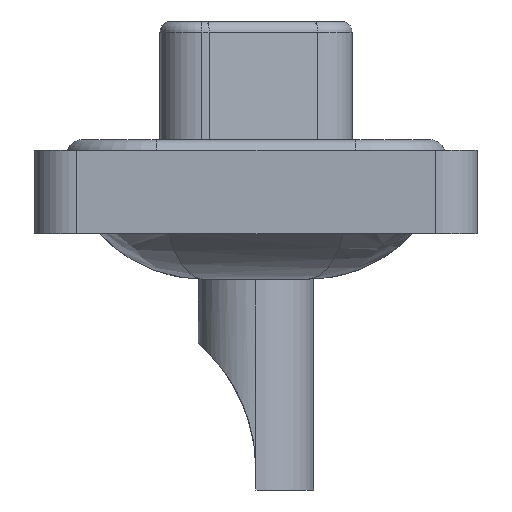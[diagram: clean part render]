
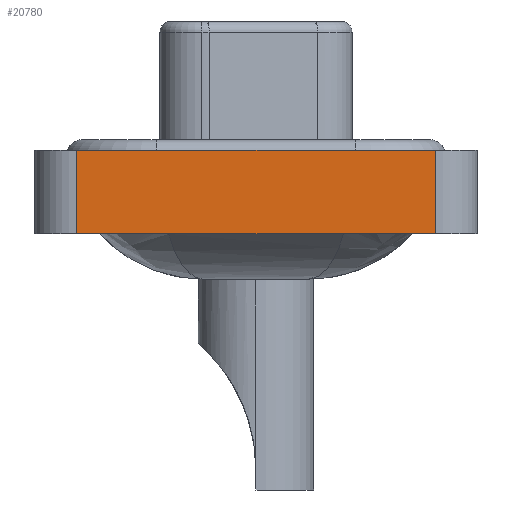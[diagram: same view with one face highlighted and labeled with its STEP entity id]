
A CAD part, left-side view. The second image highlights one B-rep face of the part: STEP entity #20780.
In plain terms, the highlighted planar face has unit normal (-1, 0, 0).
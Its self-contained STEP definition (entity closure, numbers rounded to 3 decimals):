
#815 = EDGE_LOOP ( 'NONE', ( #18101, #12877, #14945, #6495 ) ) ;
#1087 = DIRECTION ( 'NONE',  ( 0., 0., 1. ) ) ;
#1105 = VERTEX_POINT ( 'NONE', #16178 ) ;
#3852 = VERTEX_POINT ( 'NONE', #3913 ) ;
#3913 = CARTESIAN_POINT ( 'NONE',  ( -7.35, 8.55, 0.4 ) ) ;
#5101 = CARTESIAN_POINT ( 'NONE',  ( -7.35, -8.55, -3.6 ) ) ;
#5322 = DIRECTION ( 'NONE',  ( -1., 0., 0. ) ) ;
#5426 = DIRECTION ( 'NONE',  ( 0., 0., 1. ) ) ;
#6495 = ORIENTED_EDGE ( 'NONE', *, *, #6553, .T. ) ;
#6553 = EDGE_CURVE ( 'NONE', #1105, #21793, #13387, .T. ) ;
#7204 = VECTOR ( 'NONE', #14864, 1000. ) ;
#7699 = CARTESIAN_POINT ( 'NONE',  ( -7.35, 8.55, -3.6 ) ) ;
#8477 = AXIS2_PLACEMENT_3D ( 'NONE', #5101, #5322, #5426 ) ;
#9062 = CARTESIAN_POINT ( 'NONE',  ( -7.35, -8.55, 0.4 ) ) ;
#9167 = DIRECTION ( 'NONE',  ( 0., -1., 0. ) ) ;
#10273 = EDGE_CURVE ( 'NONE', #3852, #22013, #21210, .T. ) ;
#10385 = EDGE_CURVE ( 'NONE', #21793, #22013, #16330, .T. ) ;
#11111 = CARTESIAN_POINT ( 'NONE',  ( -7.35, -8.55, -3.6 ) ) ;
#11664 = DIRECTION ( 'NONE',  ( 0., -1., 0. ) ) ;
#12790 = CARTESIAN_POINT ( 'NONE',  ( -7.35, -8.55, 0.4 ) ) ;
#12877 = ORIENTED_EDGE ( 'NONE', *, *, #10273, .F. ) ;
#13387 = LINE ( 'NONE', #20286, #14992 ) ;
#14864 = DIRECTION ( 'NONE',  ( 0., 0., 1. ) ) ;
#14945 = ORIENTED_EDGE ( 'NONE', *, *, #19046, .F. ) ;
#14992 = VECTOR ( 'NONE', #11664, 1000. ) ;
#15245 = VECTOR ( 'NONE', #9167, 1000. ) ;
#15598 = VECTOR ( 'NONE', #1087, 1000. ) ;
#15669 = FACE_OUTER_BOUND ( 'NONE', #815, .T. ) ;
#15752 = CARTESIAN_POINT ( 'NONE',  ( -7.35, -8.55, -3.6 ) ) ;
#16178 = CARTESIAN_POINT ( 'NONE',  ( -7.35, 8.55, -3.6 ) ) ;
#16330 = LINE ( 'NONE', #11111, #15598 ) ;
#18101 = ORIENTED_EDGE ( 'NONE', *, *, #10385, .T. ) ;
#19046 = EDGE_CURVE ( 'NONE', #1105, #3852, #21671, .T. ) ;
#20286 = CARTESIAN_POINT ( 'NONE',  ( -7.35, -8.55, -3.6 ) ) ;
#20780 = ADVANCED_FACE ( 'NONE', ( #15669 ), #20893, .T. ) ;
#20893 = PLANE ( 'NONE',  #8477 ) ;
#21210 = LINE ( 'NONE', #9062, #15245 ) ;
#21671 = LINE ( 'NONE', #7699, #7204 ) ;
#21793 = VERTEX_POINT ( 'NONE', #15752 ) ;
#22013 = VERTEX_POINT ( 'NONE', #12790 ) ;
